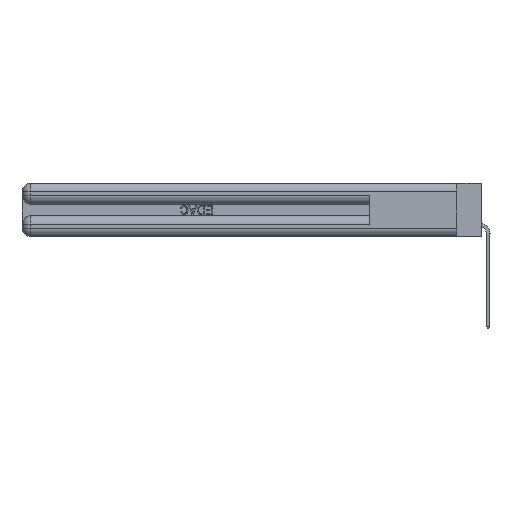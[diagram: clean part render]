
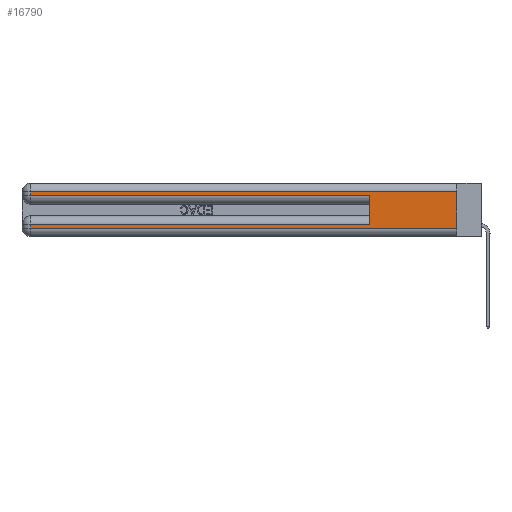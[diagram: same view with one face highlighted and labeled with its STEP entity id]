
A CAD part, left-side view. The second image highlights one B-rep face of the part: STEP entity #16790.
In plain terms, the highlighted planar face has unit normal (-1, 0, 0).
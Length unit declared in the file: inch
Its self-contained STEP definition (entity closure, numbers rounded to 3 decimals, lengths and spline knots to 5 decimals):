
#230 = PLANE ( 'NONE',  #45418 ) ;
#835 = ORIENTED_EDGE ( 'NONE', *, *, #14464, .T. ) ;
#3931 = ORIENTED_EDGE ( 'NONE', *, *, #49641, .F. ) ;
#4696 = DIRECTION ( 'NONE',  ( 1., 0., 0. ) ) ;
#4717 = VECTOR ( 'NONE', #55209, 39.37008 ) ;
#4797 = DIRECTION ( 'NONE',  ( 0., 1., 0. ) ) ;
#5332 = ORIENTED_EDGE ( 'NONE', *, *, #15791, .T. ) ;
#5760 = DIRECTION ( 'NONE',  ( 0., 0., 1. ) ) ;
#6151 = VERTEX_POINT ( 'NONE', #30854 ) ;
#8798 = EDGE_CURVE ( 'NONE', #12537, #12988, #52301, .T. ) ;
#8958 = ORIENTED_EDGE ( 'NONE', *, *, #46766, .F. ) ;
#9191 = LINE ( 'NONE', #35968, #44792 ) ;
#11578 = CARTESIAN_POINT ( 'NONE',  ( 0., 2.94, 0.285 ) ) ;
#11641 = VECTOR ( 'NONE', #20086, 39.37008 ) ;
#11761 = DIRECTION ( 'NONE',  ( 0., -1., 0. ) ) ;
#12537 = VERTEX_POINT ( 'NONE', #41443 ) ;
#12624 = EDGE_CURVE ( 'NONE', #32151, #37386, #44561, .T. ) ;
#12988 = VERTEX_POINT ( 'NONE', #22488 ) ;
#13216 = ORIENTED_EDGE ( 'NONE', *, *, #8798, .T. ) ;
#13781 = LINE ( 'NONE', #51885, #33902 ) ;
#14464 = EDGE_CURVE ( 'NONE', #20580, #26629, #44988, .T. ) ;
#14640 = VECTOR ( 'NONE', #5760, 39.37008 ) ;
#15791 = EDGE_CURVE ( 'NONE', #33246, #20580, #16714, .T. ) ;
#16714 = LINE ( 'NONE', #34221, #18733 ) ;
#16790 = ADVANCED_FACE ( 'NONE', ( #17835 ), #230, .F. ) ;
#17835 = FACE_OUTER_BOUND ( 'NONE', #45564, .T. ) ;
#18733 = VECTOR ( 'NONE', #4797, 39.37008 ) ;
#20086 = DIRECTION ( 'NONE',  ( 0., -1., 0. ) ) ;
#20580 = VERTEX_POINT ( 'NONE', #20844 ) ;
#20745 = VECTOR ( 'NONE', #22078, 39.37008 ) ;
#20844 = CARTESIAN_POINT ( 'NONE',  ( 0., 2.94, 0.31 ) ) ;
#22078 = DIRECTION ( 'NONE',  ( 0., 1., 0. ) ) ;
#22488 = CARTESIAN_POINT ( 'NONE',  ( 0., 2.94, 0.085 ) ) ;
#23704 = ORIENTED_EDGE ( 'NONE', *, *, #12624, .T. ) ;
#24158 = DIRECTION ( 'NONE',  ( 0., 0., -1. ) ) ;
#26500 = EDGE_CURVE ( 'NONE', #26629, #6151, #9191, .T. ) ;
#26629 = VERTEX_POINT ( 'NONE', #11578 ) ;
#27862 = CARTESIAN_POINT ( 'NONE',  ( 0., 0., 0.31 ) ) ;
#30360 = DIRECTION ( 'NONE',  ( 0., 0., -1. ) ) ;
#30854 = CARTESIAN_POINT ( 'NONE',  ( 0., 0.6, 0.285 ) ) ;
#32151 = VERTEX_POINT ( 'NONE', #48736 ) ;
#32800 = CARTESIAN_POINT ( 'NONE',  ( 0., 0., 0.06 ) ) ;
#33246 = VERTEX_POINT ( 'NONE', #27862 ) ;
#33818 = VECTOR ( 'NONE', #24158, 39.37008 ) ;
#33902 = VECTOR ( 'NONE', #52444, 39.37008 ) ;
#34221 = CARTESIAN_POINT ( 'NONE',  ( 0., 0., 0.31 ) ) ;
#34513 = LINE ( 'NONE', #45736, #33818 ) ;
#35968 = CARTESIAN_POINT ( 'NONE',  ( 0., 0., 0.285 ) ) ;
#37386 = VERTEX_POINT ( 'NONE', #50676 ) ;
#41443 = CARTESIAN_POINT ( 'NONE',  ( 0., 0.6, 0.085 ) ) ;
#41615 = ORIENTED_EDGE ( 'NONE', *, *, #26500, .T. ) ;
#42792 = LINE ( 'NONE', #44208, #14640 ) ;
#42913 = EDGE_CURVE ( 'NONE', #12988, #32151, #34513, .T. ) ;
#44208 = CARTESIAN_POINT ( 'NONE',  ( 0., 0.6, 0.145 ) ) ;
#44561 = LINE ( 'NONE', #32800, #11641 ) ;
#44792 = VECTOR ( 'NONE', #11761, 39.37008 ) ;
#44988 = LINE ( 'NONE', #46977, #4717 ) ;
#45418 = AXIS2_PLACEMENT_3D ( 'NONE', #47847, #4696, #30360 ) ;
#45564 = EDGE_LOOP ( 'NONE', ( #3931, #5332, #835, #41615, #8958, #13216, #51593, #23704 ) ) ;
#45736 = CARTESIAN_POINT ( 'NONE',  ( 0., 2.94, 0.37 ) ) ;
#46766 = EDGE_CURVE ( 'NONE', #12537, #6151, #42792, .T. ) ;
#46977 = CARTESIAN_POINT ( 'NONE',  ( 0., 2.94, 0.37 ) ) ;
#47847 = CARTESIAN_POINT ( 'NONE',  ( 0., 0., 0.37 ) ) ;
#48122 = CARTESIAN_POINT ( 'NONE',  ( 0., 0., 0.085 ) ) ;
#48736 = CARTESIAN_POINT ( 'NONE',  ( 0., 2.94, 0.06 ) ) ;
#49641 = EDGE_CURVE ( 'NONE', #33246, #37386, #13781, .T. ) ;
#50676 = CARTESIAN_POINT ( 'NONE',  ( 0., 0., 0.06 ) ) ;
#51593 = ORIENTED_EDGE ( 'NONE', *, *, #42913, .T. ) ;
#51885 = CARTESIAN_POINT ( 'NONE',  ( 0., 0., 0.37 ) ) ;
#52301 = LINE ( 'NONE', #48122, #20745 ) ;
#52444 = DIRECTION ( 'NONE',  ( 0., 0., -1. ) ) ;
#55209 = DIRECTION ( 'NONE',  ( 0., 0., -1. ) ) ;
